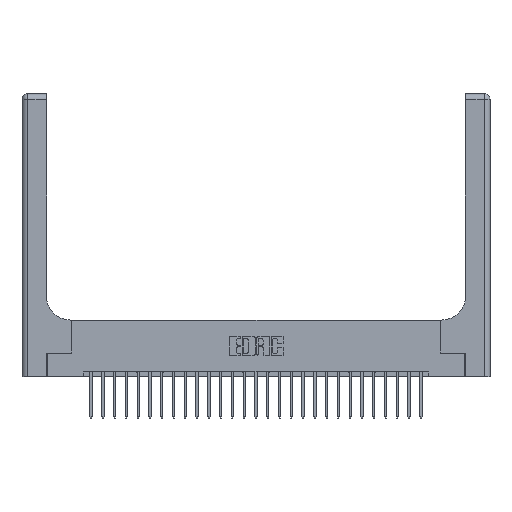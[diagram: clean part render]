
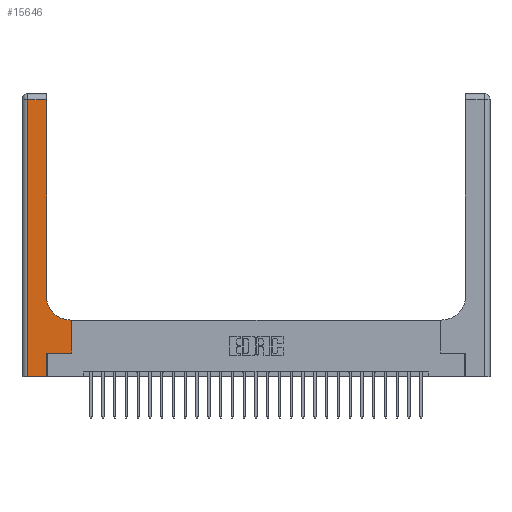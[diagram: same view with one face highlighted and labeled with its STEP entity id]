
A CAD part, top view. The second image highlights one B-rep face of the part: STEP entity #15646.
In plain terms, the highlighted planar face has unit normal (0, 0, 1).
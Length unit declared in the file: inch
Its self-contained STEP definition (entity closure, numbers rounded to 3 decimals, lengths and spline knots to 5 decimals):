
#520 = DIRECTION ( 'NONE',  ( 0., 0., -1. ) ) ;
#651 = LINE ( 'NONE', #22510, #11751 ) ;
#805 = VERTEX_POINT ( 'NONE', #25165 ) ;
#2199 = LINE ( 'NONE', #9931, #23320 ) ;
#2405 = ORIENTED_EDGE ( 'NONE', *, *, #19714, .T. ) ;
#2585 = AXIS2_PLACEMENT_3D ( 'NONE', #14773, #18629, #15036 ) ;
#2782 = DIRECTION ( 'NONE',  ( 0., 1., 0. ) ) ;
#3047 = ORIENTED_EDGE ( 'NONE', *, *, #24179, .T. ) ;
#3299 = VERTEX_POINT ( 'NONE', #4290 ) ;
#4125 = CARTESIAN_POINT ( 'NONE',  ( 0., 2.94, 0.37 ) ) ;
#4290 = CARTESIAN_POINT ( 'NONE',  ( 0.528, 0.6, 0.37 ) ) ;
#4308 = DIRECTION ( 'NONE',  ( 0., 1., 0. ) ) ;
#4549 = EDGE_LOOP ( 'NONE', ( #3047, #17853, #18306, #16718, #20469, #19016, #14374, #16604, #2405 ) ) ;
#4758 = FACE_OUTER_BOUND ( 'NONE', #4549, .T. ) ;
#5658 = LINE ( 'NONE', #11418, #20029 ) ;
#5937 = CIRCLE ( 'NONE', #2585, 0.25 ) ;
#6045 = LINE ( 'NONE', #14209, #12800 ) ;
#6069 = VERTEX_POINT ( 'NONE', #17488 ) ;
#6264 = VERTEX_POINT ( 'NONE', #20120 ) ;
#6295 = CARTESIAN_POINT ( 'NONE',  ( 0.26, 2.94, 0.37 ) ) ;
#6833 = VERTEX_POINT ( 'NONE', #18614 ) ;
#6902 = CARTESIAN_POINT ( 'NONE',  ( 0.265, 0.25, 0.37 ) ) ;
#8363 = EDGE_CURVE ( 'NONE', #6833, #3299, #21063, .T. ) ;
#8940 = VERTEX_POINT ( 'NONE', #6295 ) ;
#9358 = DIRECTION ( 'NONE',  ( 1., 0., 0. ) ) ;
#9759 = CARTESIAN_POINT ( 'NONE',  ( 0., 0., 0.37 ) ) ;
#9803 = DIRECTION ( 'NONE',  ( -1., 0., 0. ) ) ;
#9931 = CARTESIAN_POINT ( 'NONE',  ( 0.06, 3., 0.37 ) ) ;
#10070 = CARTESIAN_POINT ( 'NONE',  ( 0.51, 0.6, 0.37 ) ) ;
#10356 = DIRECTION ( 'NONE',  ( 0., 1., 0. ) ) ;
#10537 = EDGE_CURVE ( 'NONE', #805, #6069, #11623, .T. ) ;
#11418 = CARTESIAN_POINT ( 'NONE',  ( 0.26, 0.6, 0.37 ) ) ;
#11623 = LINE ( 'NONE', #9759, #11671 ) ;
#11671 = VECTOR ( 'NONE', #9358, 39.37008 ) ;
#11751 = VECTOR ( 'NONE', #10356, 39.37008 ) ;
#12728 = EDGE_CURVE ( 'NONE', #6069, #19257, #651, .T. ) ;
#12800 = VECTOR ( 'NONE', #4308, 39.37008 ) ;
#13108 = VECTOR ( 'NONE', #25801, 39.37008 ) ;
#13626 = CARTESIAN_POINT ( 'NONE',  ( 0.26, 0.85, 0.37 ) ) ;
#14209 = CARTESIAN_POINT ( 'NONE',  ( 0.26, 3., 0.37 ) ) ;
#14299 = LINE ( 'NONE', #4125, #25631 ) ;
#14309 = VECTOR ( 'NONE', #2782, 39.37008 ) ;
#14354 = DIRECTION ( 'NONE',  ( 0., -1., 0. ) ) ;
#14374 = ORIENTED_EDGE ( 'NONE', *, *, #8363, .T. ) ;
#14669 = EDGE_CURVE ( 'NONE', #19257, #6833, #22067, .T. ) ;
#14773 = CARTESIAN_POINT ( 'NONE',  ( 0.51, 0.85, 0.37 ) ) ;
#15036 = DIRECTION ( 'NONE',  ( 1., 0., 0. ) ) ;
#15563 = CARTESIAN_POINT ( 'NONE',  ( 0.265, 0.25, 0.37 ) ) ;
#15646 = ADVANCED_FACE ( 'NONE', ( #4758 ), #23043, .F. ) ;
#16027 = EDGE_CURVE ( 'NONE', #6264, #805, #2199, .T. ) ;
#16604 = ORIENTED_EDGE ( 'NONE', *, *, #24111, .T. ) ;
#16718 = ORIENTED_EDGE ( 'NONE', *, *, #10537, .T. ) ;
#17067 = CARTESIAN_POINT ( 'NONE',  ( 0., 3., 0.37 ) ) ;
#17488 = CARTESIAN_POINT ( 'NONE',  ( 0.265, 0., 0.37 ) ) ;
#17853 = ORIENTED_EDGE ( 'NONE', *, *, #21743, .T. ) ;
#18306 = ORIENTED_EDGE ( 'NONE', *, *, #16027, .T. ) ;
#18614 = CARTESIAN_POINT ( 'NONE',  ( 0.528, 0.25, 0.37 ) ) ;
#18629 = DIRECTION ( 'NONE',  ( 0., 0., -1. ) ) ;
#19016 = ORIENTED_EDGE ( 'NONE', *, *, #14669, .T. ) ;
#19257 = VERTEX_POINT ( 'NONE', #6902 ) ;
#19453 = CARTESIAN_POINT ( 'NONE',  ( 0.528, 0.25, 0.37 ) ) ;
#19533 = AXIS2_PLACEMENT_3D ( 'NONE', #17067, #520, #21326 ) ;
#19714 = EDGE_CURVE ( 'NONE', #20909, #24937, #5937, .T. ) ;
#20029 = VECTOR ( 'NONE', #9803, 39.37008 ) ;
#20120 = CARTESIAN_POINT ( 'NONE',  ( 0.06, 2.94, 0.37 ) ) ;
#20469 = ORIENTED_EDGE ( 'NONE', *, *, #12728, .T. ) ;
#20909 = VERTEX_POINT ( 'NONE', #10070 ) ;
#21063 = LINE ( 'NONE', #19453, #14309 ) ;
#21326 = DIRECTION ( 'NONE',  ( -1., 0., 0. ) ) ;
#21743 = EDGE_CURVE ( 'NONE', #8940, #6264, #14299, .T. ) ;
#22067 = LINE ( 'NONE', #15563, #13108 ) ;
#22510 = CARTESIAN_POINT ( 'NONE',  ( 0.265, 0., 0.37 ) ) ;
#23043 = PLANE ( 'NONE',  #19533 ) ;
#23320 = VECTOR ( 'NONE', #14354, 39.37008 ) ;
#24111 = EDGE_CURVE ( 'NONE', #3299, #20909, #5658, .T. ) ;
#24179 = EDGE_CURVE ( 'NONE', #24937, #8940, #6045, .T. ) ;
#24407 = DIRECTION ( 'NONE',  ( -1., 0., 0. ) ) ;
#24937 = VERTEX_POINT ( 'NONE', #13626 ) ;
#25165 = CARTESIAN_POINT ( 'NONE',  ( 0.06, 0., 0.37 ) ) ;
#25631 = VECTOR ( 'NONE', #24407, 39.37008 ) ;
#25801 = DIRECTION ( 'NONE',  ( 1., 0., 0. ) ) ;
